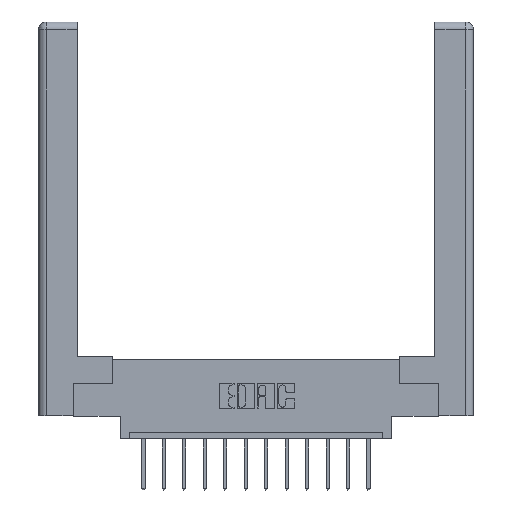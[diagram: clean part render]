
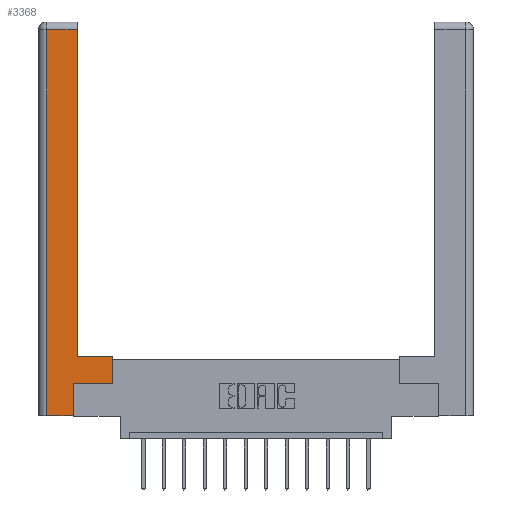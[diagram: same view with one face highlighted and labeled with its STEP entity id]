
A CAD part, top view. The second image highlights one B-rep face of the part: STEP entity #3368.
In plain terms, the highlighted planar face has unit normal (0, 0, 1).
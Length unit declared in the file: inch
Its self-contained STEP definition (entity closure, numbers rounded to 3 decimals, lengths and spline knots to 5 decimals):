
#15 = CARTESIAN_POINT ( 'NONE',  ( 0.0615, 2.94, 0. ) ) ;
#206 = VECTOR ( 'NONE', #11205, 39.37008 ) ;
#416 = EDGE_CURVE ( 'NONE', #13374, #6505, #8567, .T. ) ;
#669 = DIRECTION ( 'NONE',  ( 0., -1., 0. ) ) ;
#778 = CARTESIAN_POINT ( 'NONE',  ( 0.0615, 0., 0. ) ) ;
#1166 = ORIENTED_EDGE ( 'NONE', *, *, #6911, .T. ) ;
#1607 = VECTOR ( 'NONE', #1655, 39.37008 ) ;
#1655 = DIRECTION ( 'NONE',  ( -1., 0., 0. ) ) ;
#1660 = CARTESIAN_POINT ( 'NONE',  ( 0.295, 3., 0. ) ) ;
#1693 = VECTOR ( 'NONE', #12960, 39.37008 ) ;
#2382 = CARTESIAN_POINT ( 'NONE',  ( 0., 0., 0. ) ) ;
#2425 = EDGE_CURVE ( 'NONE', #12639, #9498, #13941, .T. ) ;
#2634 = DIRECTION ( 'NONE',  ( 1., 0., 0. ) ) ;
#2764 = ORIENTED_EDGE ( 'NONE', *, *, #5236, .T. ) ;
#2922 = VERTEX_POINT ( 'NONE', #6871 ) ;
#3368 = ADVANCED_FACE ( 'NONE', ( #13908 ), #8339, .F. ) ;
#3746 = CARTESIAN_POINT ( 'NONE',  ( 0.295, 2.94, 0. ) ) ;
#3887 = CARTESIAN_POINT ( 'NONE',  ( 0.265, 0.245, 0. ) ) ;
#3990 = CARTESIAN_POINT ( 'NONE',  ( 0.295, 0.45, 0. ) ) ;
#4074 = EDGE_CURVE ( 'NONE', #8875, #12361, #5214, .T. ) ;
#4236 = LINE ( 'NONE', #14914, #11777 ) ;
#4328 = DIRECTION ( 'NONE',  ( 0., 1., 0. ) ) ;
#4781 = VECTOR ( 'NONE', #669, 39.37008 ) ;
#5214 = LINE ( 'NONE', #1660, #6929 ) ;
#5220 = EDGE_CURVE ( 'NONE', #14406, #8875, #12143, .T. ) ;
#5236 = EDGE_CURVE ( 'NONE', #6505, #12639, #4236, .T. ) ;
#5388 = EDGE_CURVE ( 'NONE', #2922, #14406, #8590, .T. ) ;
#5848 = VECTOR ( 'NONE', #2634, 39.37008 ) ;
#6505 = VERTEX_POINT ( 'NONE', #7090 ) ;
#6804 = ORIENTED_EDGE ( 'NONE', *, *, #7750, .T. ) ;
#6871 = CARTESIAN_POINT ( 'NONE',  ( 0.565, 0.245, 0. ) ) ;
#6911 = EDGE_CURVE ( 'NONE', #9498, #2922, #11520, .T. ) ;
#6929 = VECTOR ( 'NONE', #15084, 39.37008 ) ;
#7090 = CARTESIAN_POINT ( 'NONE',  ( 0.0615, 0., 0. ) ) ;
#7534 = CARTESIAN_POINT ( 'NONE',  ( 0.565, 0.245, 0. ) ) ;
#7569 = ORIENTED_EDGE ( 'NONE', *, *, #416, .T. ) ;
#7716 = DIRECTION ( 'NONE',  ( 1., 0., 0. ) ) ;
#7750 = EDGE_CURVE ( 'NONE', #12361, #13374, #9605, .T. ) ;
#7833 = VECTOR ( 'NONE', #4328, 39.37008 ) ;
#8339 = PLANE ( 'NONE',  #9894 ) ;
#8567 = LINE ( 'NONE', #778, #4781 ) ;
#8590 = LINE ( 'NONE', #11392, #7833 ) ;
#8851 = ORIENTED_EDGE ( 'NONE', *, *, #5220, .T. ) ;
#8875 = VERTEX_POINT ( 'NONE', #3990 ) ;
#9297 = EDGE_LOOP ( 'NONE', ( #12212, #6804, #7569, #2764, #15364, #1166, #14251, #8851 ) ) ;
#9498 = VERTEX_POINT ( 'NONE', #9692 ) ;
#9605 = LINE ( 'NONE', #14130, #1693 ) ;
#9640 = DIRECTION ( 'NONE',  ( -1., 0., 0. ) ) ;
#9692 = CARTESIAN_POINT ( 'NONE',  ( 0.265, 0.245, 0. ) ) ;
#9894 = AXIS2_PLACEMENT_3D ( 'NONE', #2382, #11892, #9640 ) ;
#11205 = DIRECTION ( 'NONE',  ( 0., 1., 0. ) ) ;
#11392 = CARTESIAN_POINT ( 'NONE',  ( 0.565, 0.45, 0. ) ) ;
#11520 = LINE ( 'NONE', #7534, #5848 ) ;
#11612 = CARTESIAN_POINT ( 'NONE',  ( 0.265, 0., 0. ) ) ;
#11777 = VECTOR ( 'NONE', #7716, 39.37008 ) ;
#11892 = DIRECTION ( 'NONE',  ( 0., 0., -1. ) ) ;
#12143 = LINE ( 'NONE', #12543, #1607 ) ;
#12212 = ORIENTED_EDGE ( 'NONE', *, *, #4074, .T. ) ;
#12361 = VERTEX_POINT ( 'NONE', #3746 ) ;
#12543 = CARTESIAN_POINT ( 'NONE',  ( 0.295, 0.45, 0. ) ) ;
#12639 = VERTEX_POINT ( 'NONE', #11612 ) ;
#12960 = DIRECTION ( 'NONE',  ( -1., 0., 0. ) ) ;
#13374 = VERTEX_POINT ( 'NONE', #15 ) ;
#13908 = FACE_OUTER_BOUND ( 'NONE', #9297, .T. ) ;
#13941 = LINE ( 'NONE', #3887, #206 ) ;
#14130 = CARTESIAN_POINT ( 'NONE',  ( 0.0615, 2.94, 0. ) ) ;
#14251 = ORIENTED_EDGE ( 'NONE', *, *, #5388, .T. ) ;
#14406 = VERTEX_POINT ( 'NONE', #15026 ) ;
#14914 = CARTESIAN_POINT ( 'NONE',  ( 0.265, 0., 0. ) ) ;
#15026 = CARTESIAN_POINT ( 'NONE',  ( 0.565, 0.45, 0. ) ) ;
#15084 = DIRECTION ( 'NONE',  ( 0., 1., 0. ) ) ;
#15364 = ORIENTED_EDGE ( 'NONE', *, *, #2425, .T. ) ;
